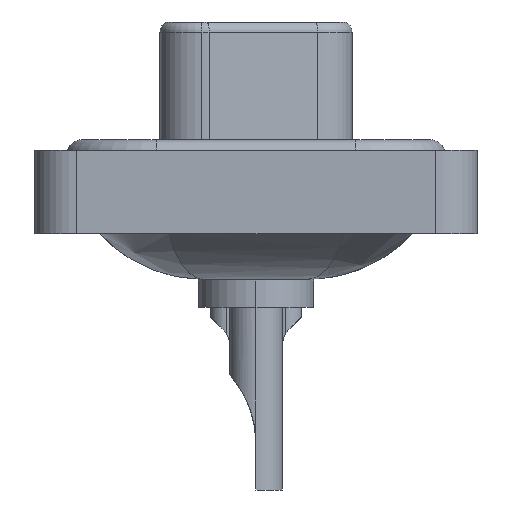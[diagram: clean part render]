
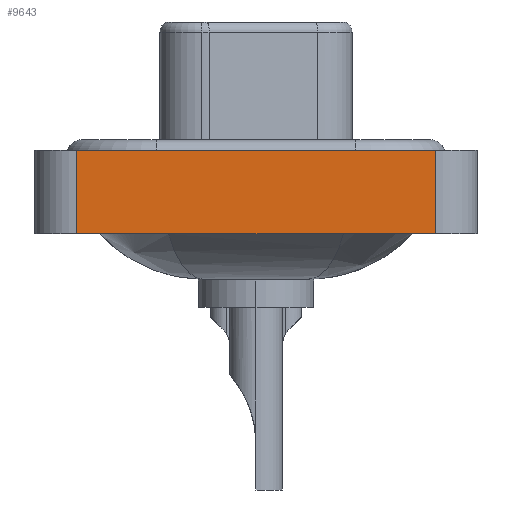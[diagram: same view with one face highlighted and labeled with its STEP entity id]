
A CAD part, left-side view. The second image highlights one B-rep face of the part: STEP entity #9643.
In plain terms, the highlighted planar face has unit normal (-1, 0, 0).
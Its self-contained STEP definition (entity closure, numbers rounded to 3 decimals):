
#395 = VECTOR ( 'NONE', #18981, 1000. ) ;
#606 = CARTESIAN_POINT ( 'NONE',  ( -7.3, -8.55, -3.6 ) ) ;
#1483 = CARTESIAN_POINT ( 'NONE',  ( -7.3, 8.55, 0.4 ) ) ;
#2245 = DIRECTION ( 'NONE',  ( 0., -1., 0. ) ) ;
#2477 = ORIENTED_EDGE ( 'NONE', *, *, #10019, .F. ) ;
#3882 = CARTESIAN_POINT ( 'NONE',  ( -7.3, 8.55, -3.6 ) ) ;
#5079 = EDGE_LOOP ( 'NONE', ( #9315, #2477, #10039, #17372 ) ) ;
#6905 = DIRECTION ( 'NONE',  ( 0., 0., 1. ) ) ;
#6948 = CARTESIAN_POINT ( 'NONE',  ( -7.3, -8.55, 0.4 ) ) ;
#7551 = CARTESIAN_POINT ( 'NONE',  ( -7.3, 8.55, -3.6 ) ) ;
#8167 = LINE ( 'NONE', #6948, #14696 ) ;
#8758 = DIRECTION ( 'NONE',  ( 0., 0., 1. ) ) ;
#9083 = CARTESIAN_POINT ( 'NONE',  ( -7.3, -8.55, 0.4 ) ) ;
#9315 = ORIENTED_EDGE ( 'NONE', *, *, #15226, .T. ) ;
#9631 = VERTEX_POINT ( 'NONE', #3882 ) ;
#9643 = ADVANCED_FACE ( 'NONE', ( #15907 ), #16006, .T. ) ;
#10019 = EDGE_CURVE ( 'NONE', #18638, #13377, #8167, .T. ) ;
#10039 = ORIENTED_EDGE ( 'NONE', *, *, #16450, .F. ) ;
#11245 = LINE ( 'NONE', #14359, #11959 ) ;
#11959 = VECTOR ( 'NONE', #6905, 1000. ) ;
#13377 = VERTEX_POINT ( 'NONE', #9083 ) ;
#14330 = EDGE_CURVE ( 'NONE', #9631, #18810, #14368, .T. ) ;
#14359 = CARTESIAN_POINT ( 'NONE',  ( -7.3, -8.55, -3.6 ) ) ;
#14368 = LINE ( 'NONE', #606, #395 ) ;
#14518 = CARTESIAN_POINT ( 'NONE',  ( -7.3, -8.55, -3.6 ) ) ;
#14696 = VECTOR ( 'NONE', #2245, 1000. ) ;
#14719 = DIRECTION ( 'NONE',  ( 0., 0., 1. ) ) ;
#15226 = EDGE_CURVE ( 'NONE', #18810, #13377, #11245, .T. ) ;
#15907 = FACE_OUTER_BOUND ( 'NONE', #5079, .T. ) ;
#16006 = PLANE ( 'NONE',  #19785 ) ;
#16111 = DIRECTION ( 'NONE',  ( -1., 0., 0. ) ) ;
#16450 = EDGE_CURVE ( 'NONE', #9631, #18638, #18189, .T. ) ;
#17364 = VECTOR ( 'NONE', #8758, 1000. ) ;
#17372 = ORIENTED_EDGE ( 'NONE', *, *, #14330, .T. ) ;
#18189 = LINE ( 'NONE', #7551, #17364 ) ;
#18638 = VERTEX_POINT ( 'NONE', #1483 ) ;
#18810 = VERTEX_POINT ( 'NONE', #14518 ) ;
#18981 = DIRECTION ( 'NONE',  ( 0., -1., 0. ) ) ;
#19043 = CARTESIAN_POINT ( 'NONE',  ( -7.3, -8.55, -3.6 ) ) ;
#19785 = AXIS2_PLACEMENT_3D ( 'NONE', #19043, #16111, #14719 ) ;
